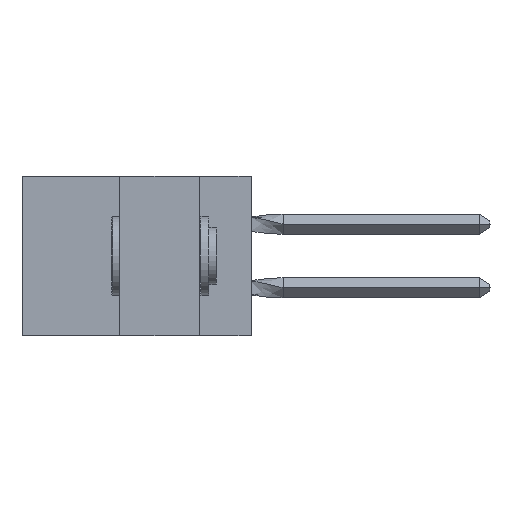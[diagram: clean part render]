
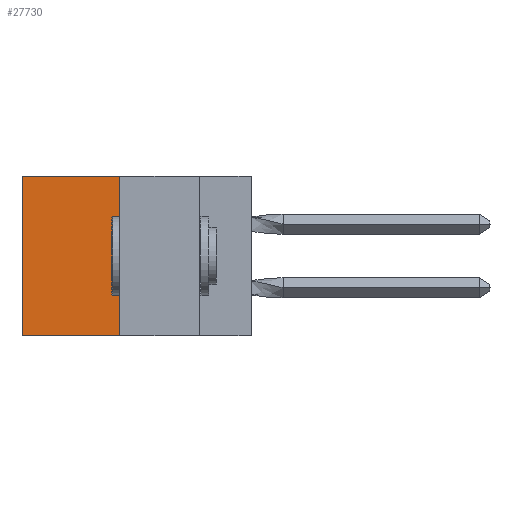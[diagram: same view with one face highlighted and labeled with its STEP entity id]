
A CAD part, left-side view. The second image highlights one B-rep face of the part: STEP entity #27730.
In plain terms, the highlighted planar face has unit normal (-1, 0, 0).
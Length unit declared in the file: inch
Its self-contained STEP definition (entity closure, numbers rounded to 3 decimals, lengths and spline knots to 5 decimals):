
#846 = VERTEX_POINT ( 'NONE', #30279 ) ;
#3496 = VERTEX_POINT ( 'NONE', #29026 ) ;
#3587 = VECTOR ( 'NONE', #7024, 39.37008 ) ;
#4170 = DIRECTION ( 'NONE',  ( 0., 0., -1. ) ) ;
#5488 = LINE ( 'NONE', #28185, #3587 ) ;
#5870 = CARTESIAN_POINT ( 'NONE',  ( 0.305, 0.413, -0.5 ) ) ;
#6133 = CARTESIAN_POINT ( 'NONE',  ( 0.305, 0.413, -0.5 ) ) ;
#6269 = DIRECTION ( 'NONE',  ( 0., 1., 0. ) ) ;
#7024 = DIRECTION ( 'NONE',  ( 0., 1., 0. ) ) ;
#8327 = VECTOR ( 'NONE', #4170, 39.37008 ) ;
#9513 = EDGE_CURVE ( 'NONE', #33992, #29974, #26307, .T. ) ;
#10665 = LINE ( 'NONE', #5870, #29257 ) ;
#10763 = DIRECTION ( 'NONE',  ( 1., 0., 0. ) ) ;
#12958 = EDGE_CURVE ( 'NONE', #33992, #846, #5488, .T. ) ;
#15938 = FACE_OUTER_BOUND ( 'NONE', #38976, .T. ) ;
#16951 = CARTESIAN_POINT ( 'NONE',  ( 0.305, 0.413, -0.5 ) ) ;
#17475 = PLANE ( 'NONE',  #26078 ) ;
#19153 = CARTESIAN_POINT ( 'NONE',  ( 0.305, 0.413, -0.5 ) ) ;
#20006 = ORIENTED_EDGE ( 'NONE', *, *, #12958, .T. ) ;
#21625 = DIRECTION ( 'NONE',  ( 0., 0., -1. ) ) ;
#22401 = ORIENTED_EDGE ( 'NONE', *, *, #9513, .F. ) ;
#23677 = ORIENTED_EDGE ( 'NONE', *, *, #32888, .T. ) ;
#25832 = EDGE_CURVE ( 'NONE', #29974, #3496, #10665, .T. ) ;
#26078 = AXIS2_PLACEMENT_3D ( 'NONE', #16951, #10763, #29228 ) ;
#26307 = LINE ( 'NONE', #19153, #31034 ) ;
#27730 = ADVANCED_FACE ( 'NONE', ( #15938 ), #17475, .F. ) ;
#28185 = CARTESIAN_POINT ( 'NONE',  ( 0.305, 0.413, 0. ) ) ;
#28400 = CARTESIAN_POINT ( 'NONE',  ( 0.305, 0.72, -0.5 ) ) ;
#28431 = ORIENTED_EDGE ( 'NONE', *, *, #25832, .F. ) ;
#29026 = CARTESIAN_POINT ( 'NONE',  ( 0.305, 0.72, -0.5 ) ) ;
#29228 = DIRECTION ( 'NONE',  ( 0., 0., -1. ) ) ;
#29257 = VECTOR ( 'NONE', #6269, 39.37008 ) ;
#29974 = VERTEX_POINT ( 'NONE', #6133 ) ;
#30279 = CARTESIAN_POINT ( 'NONE',  ( 0.305, 0.72, 0. ) ) ;
#31034 = VECTOR ( 'NONE', #21625, 39.37008 ) ;
#32888 = EDGE_CURVE ( 'NONE', #846, #3496, #37842, .T. ) ;
#33992 = VERTEX_POINT ( 'NONE', #34377 ) ;
#34377 = CARTESIAN_POINT ( 'NONE',  ( 0.305, 0.413, 0. ) ) ;
#37842 = LINE ( 'NONE', #28400, #8327 ) ;
#38976 = EDGE_LOOP ( 'NONE', ( #23677, #28431, #22401, #20006 ) ) ;
